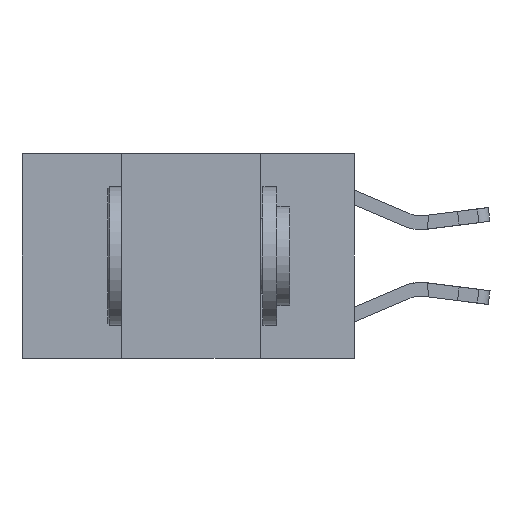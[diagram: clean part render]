
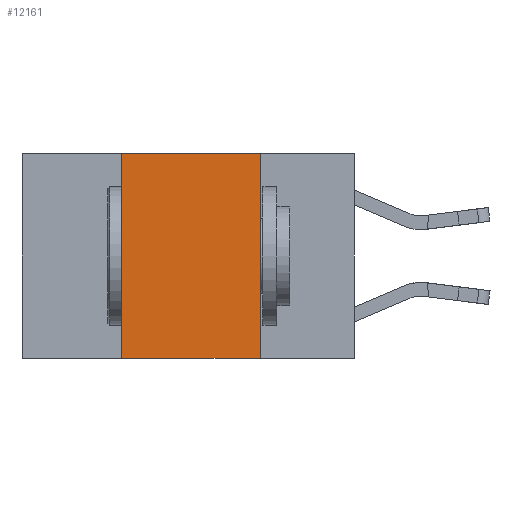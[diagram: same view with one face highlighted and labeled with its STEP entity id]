
A CAD part, left-side view. The second image highlights one B-rep face of the part: STEP entity #12161.
In plain terms, the highlighted planar face has unit normal (-1, 0, 0).
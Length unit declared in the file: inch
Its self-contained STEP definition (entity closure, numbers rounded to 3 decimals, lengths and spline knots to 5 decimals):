
#195 = ORIENTED_EDGE ( 'NONE', *, *, #11514, .F. ) ;
#818 = DIRECTION ( 'NONE',  ( 0., 0., 1. ) ) ;
#2468 = VERTEX_POINT ( 'NONE', #14005 ) ;
#2821 = DIRECTION ( 'NONE',  ( 0., -1., 0. ) ) ;
#3109 = LINE ( 'NONE', #19460, #12324 ) ;
#3312 = EDGE_CURVE ( 'NONE', #7094, #18363, #5321, .T. ) ;
#3866 = VECTOR ( 'NONE', #2821, 39.37008 ) ;
#4107 = EDGE_CURVE ( 'NONE', #18363, #21346, #8169, .T. ) ;
#5321 = LINE ( 'NONE', #11787, #10220 ) ;
#6093 = CARTESIAN_POINT ( 'NONE',  ( 0., 0.6, 0. ) ) ;
#7094 = VERTEX_POINT ( 'NONE', #19916 ) ;
#7236 = EDGE_LOOP ( 'NONE', ( #195, #19873, #20450, #16158 ) ) ;
#7803 = CARTESIAN_POINT ( 'NONE',  ( 0., 0.42, 0. ) ) ;
#7973 = PLANE ( 'NONE',  #16259 ) ;
#8169 = LINE ( 'NONE', #8297, #3866 ) ;
#8297 = CARTESIAN_POINT ( 'NONE',  ( 0., 0.6, 0. ) ) ;
#8649 = FACE_OUTER_BOUND ( 'NONE', #7236, .T. ) ;
#10220 = VECTOR ( 'NONE', #818, 39.37008 ) ;
#11514 = EDGE_CURVE ( 'NONE', #21346, #2468, #12723, .T. ) ;
#11671 = DIRECTION ( 'NONE',  ( 0., 0., -1. ) ) ;
#11787 = CARTESIAN_POINT ( 'NONE',  ( 0., 0.42, 0. ) ) ;
#12127 = VECTOR ( 'NONE', #18298, 39.37008 ) ;
#12161 = ADVANCED_FACE ( 'NONE', ( #8649 ), #7973, .F. ) ;
#12324 = VECTOR ( 'NONE', #19544, 39.37008 ) ;
#12723 = LINE ( 'NONE', #16428, #12127 ) ;
#13146 = CARTESIAN_POINT ( 'NONE',  ( 0., 0.17, 0. ) ) ;
#14005 = CARTESIAN_POINT ( 'NONE',  ( 0., 0.17, -0.37 ) ) ;
#14319 = EDGE_CURVE ( 'NONE', #7094, #2468, #3109, .T. ) ;
#16158 = ORIENTED_EDGE ( 'NONE', *, *, #14319, .T. ) ;
#16259 = AXIS2_PLACEMENT_3D ( 'NONE', #6093, #22767, #11671 ) ;
#16428 = CARTESIAN_POINT ( 'NONE',  ( 0., 0.17, 0. ) ) ;
#18298 = DIRECTION ( 'NONE',  ( 0., 0., -1. ) ) ;
#18363 = VERTEX_POINT ( 'NONE', #7803 ) ;
#19460 = CARTESIAN_POINT ( 'NONE',  ( 0., 0.6, -0.37 ) ) ;
#19544 = DIRECTION ( 'NONE',  ( 0., -1., 0. ) ) ;
#19873 = ORIENTED_EDGE ( 'NONE', *, *, #4107, .F. ) ;
#19916 = CARTESIAN_POINT ( 'NONE',  ( 0., 0.42, -0.37 ) ) ;
#20450 = ORIENTED_EDGE ( 'NONE', *, *, #3312, .F. ) ;
#21346 = VERTEX_POINT ( 'NONE', #13146 ) ;
#22767 = DIRECTION ( 'NONE',  ( 1., 0., 0. ) ) ;
